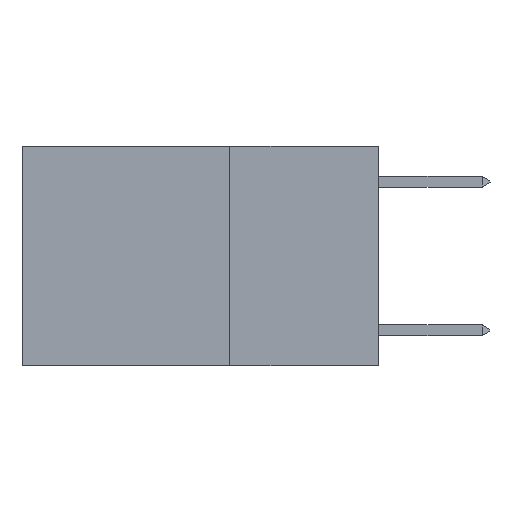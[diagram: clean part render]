
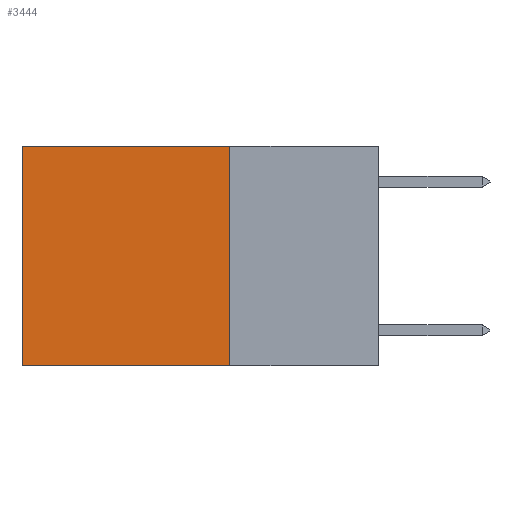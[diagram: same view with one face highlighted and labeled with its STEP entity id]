
A CAD part, left-side view. The second image highlights one B-rep face of the part: STEP entity #3444.
In plain terms, the highlighted planar face has unit normal (-1, 0, 0).
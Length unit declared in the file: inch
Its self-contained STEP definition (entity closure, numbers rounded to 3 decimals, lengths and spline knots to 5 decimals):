
#266 = DIRECTION ( 'NONE',  ( 0., 0., -1. ) ) ;
#383 = CARTESIAN_POINT ( 'NONE',  ( 0.2625, 0.25, 0. ) ) ;
#468 = EDGE_CURVE ( 'NONE', #6336, #537, #6144, .T. ) ;
#537 = VERTEX_POINT ( 'NONE', #8176 ) ;
#604 = CARTESIAN_POINT ( 'NONE',  ( 0.2625, 0.6, 0. ) ) ;
#621 = AXIS2_PLACEMENT_3D ( 'NONE', #5917, #6010, #7174 ) ;
#1181 = CARTESIAN_POINT ( 'NONE',  ( 0.2625, 0.25, -0.37 ) ) ;
#1224 = DIRECTION ( 'NONE',  ( 0., 1., 0. ) ) ;
#1526 = EDGE_CURVE ( 'NONE', #3858, #7228, #3045, .T. ) ;
#1598 = CARTESIAN_POINT ( 'NONE',  ( 0.2625, 0.25, 0. ) ) ;
#2116 = ORIENTED_EDGE ( 'NONE', *, *, #1526, .F. ) ;
#2756 = ORIENTED_EDGE ( 'NONE', *, *, #468, .T. ) ;
#2839 = CARTESIAN_POINT ( 'NONE',  ( 0.2625, 0.6, 0. ) ) ;
#2874 = LINE ( 'NONE', #1598, #3486 ) ;
#2896 = VECTOR ( 'NONE', #5008, 39.37008 ) ;
#2954 = CARTESIAN_POINT ( 'NONE',  ( 0.2625, 0.25, 0. ) ) ;
#3045 = LINE ( 'NONE', #383, #2896 ) ;
#3263 = PLANE ( 'NONE',  #621 ) ;
#3444 = ADVANCED_FACE ( 'NONE', ( #4120 ), #3263, .F. ) ;
#3452 = VECTOR ( 'NONE', #266, 39.37008 ) ;
#3486 = VECTOR ( 'NONE', #8083, 39.37008 ) ;
#3858 = VERTEX_POINT ( 'NONE', #2954 ) ;
#4120 = FACE_OUTER_BOUND ( 'NONE', #7518, .T. ) ;
#4266 = EDGE_CURVE ( 'NONE', #3858, #6336, #2874, .T. ) ;
#4539 = LINE ( 'NONE', #7634, #5581 ) ;
#5008 = DIRECTION ( 'NONE',  ( 0., 0., -1. ) ) ;
#5581 = VECTOR ( 'NONE', #1224, 39.37008 ) ;
#5909 = EDGE_CURVE ( 'NONE', #7228, #537, #4539, .T. ) ;
#5917 = CARTESIAN_POINT ( 'NONE',  ( 0.2625, 0.25, 0. ) ) ;
#6010 = DIRECTION ( 'NONE',  ( 1., 0., 0. ) ) ;
#6144 = LINE ( 'NONE', #2839, #3452 ) ;
#6336 = VERTEX_POINT ( 'NONE', #604 ) ;
#6443 = ORIENTED_EDGE ( 'NONE', *, *, #4266, .T. ) ;
#6724 = ORIENTED_EDGE ( 'NONE', *, *, #5909, .F. ) ;
#7174 = DIRECTION ( 'NONE',  ( 0., 0., -1. ) ) ;
#7228 = VERTEX_POINT ( 'NONE', #1181 ) ;
#7518 = EDGE_LOOP ( 'NONE', ( #2756, #6724, #2116, #6443 ) ) ;
#7634 = CARTESIAN_POINT ( 'NONE',  ( 0.2625, 0.25, -0.37 ) ) ;
#8083 = DIRECTION ( 'NONE',  ( 0., 1., 0. ) ) ;
#8176 = CARTESIAN_POINT ( 'NONE',  ( 0.2625, 0.6, -0.37 ) ) ;
